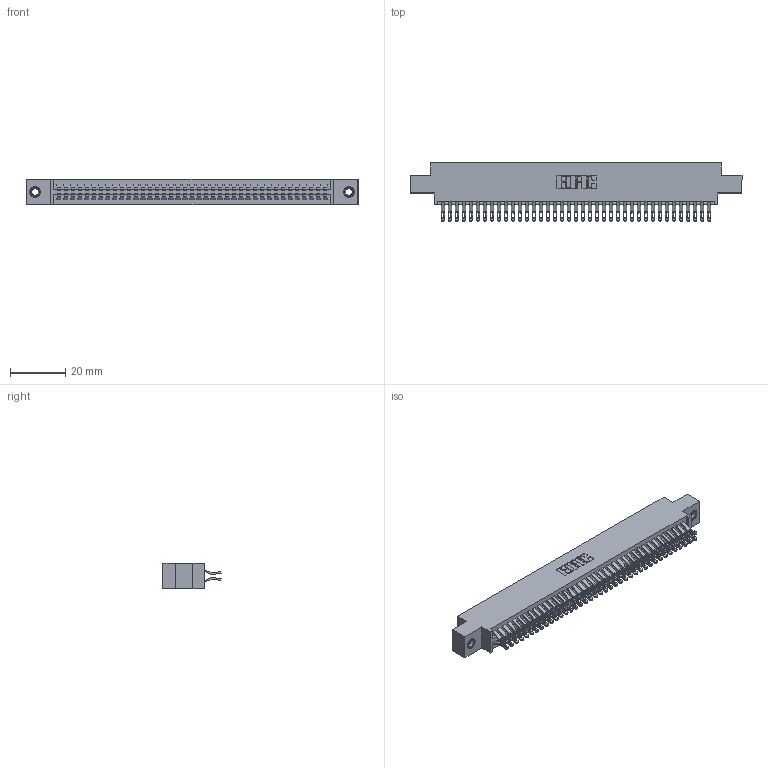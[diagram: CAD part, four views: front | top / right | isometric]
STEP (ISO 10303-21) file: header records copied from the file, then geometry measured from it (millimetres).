
FILE_DESCRIPTION (( 'STEP AP203' ), '1' );
FILE_NAME ('345-078-555-807.STEP', '2019-10-31T16:38:00', ( '' ), ( '' ), 'SwSTEP 2.0', 'SolidWorks 2016', '' );
FILE_SCHEMA (( 'CONFIG_CONTROL_DESIGN' ));
Length unit declared in the file: inch
Products named in the file (4): 345 Part_0.170 Offset - 0.156 Dia-TI; 345-250-001_345-250-005-103; 345-078-555-807; 345-292-001_555 Tail
Assembly tree (81 placements, depth 2):
  345-078-555-807
    345 Part_0.170 Offset - 0.156 Dia-TI
    345-292-001_555 Tail  x78
    345-250-001_345-250-005-103  x2
Bounding box: 120.27 x 21.13 x 9.4 mm (x, y, z)
Volume: 11754.5 mm3; surface area: 18275.3 mm2
Topology: 81 solids, 81 shells, 4558 faces, 14295 edges, 9522 vertices
Faces by surface type: plane 2534, cylinder 2008, cone 12, torus 4
Entity records: 32648 total; most frequent: CARTESIAN_POINT 5493, ORIENTED_EDGE 5390, DIRECTION 4841, EDGE_CURVE 2695, VECTOR 2367, LINE 2367, VERTEX_POINT 1792, AXIS2_PLACEMENT_3D 1237
